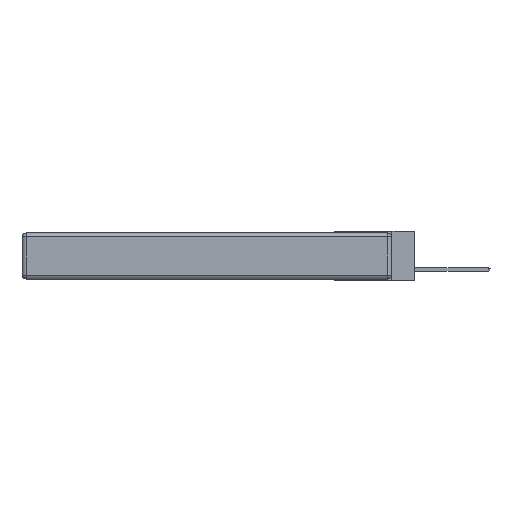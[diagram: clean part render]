
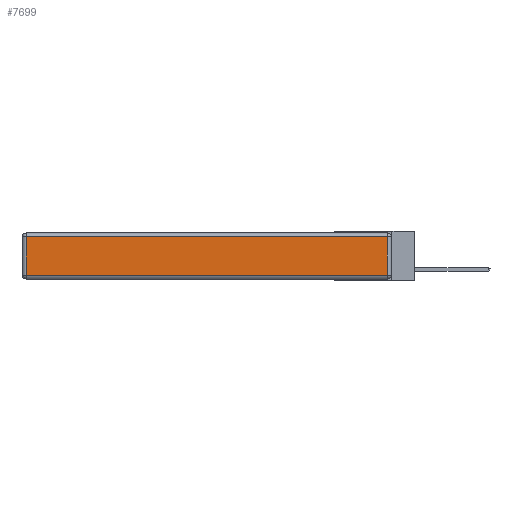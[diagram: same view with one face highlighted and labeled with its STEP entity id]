
A CAD part, left-side view. The second image highlights one B-rep face of the part: STEP entity #7699.
In plain terms, the highlighted planar face has unit normal (-1, 0, 0).
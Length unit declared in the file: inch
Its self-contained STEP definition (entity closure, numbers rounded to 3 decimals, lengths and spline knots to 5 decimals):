
#28 = VERTEX_POINT ( 'NONE', #29723 ) ;
#1536 = CARTESIAN_POINT ( 'NONE',  ( 0., 0.03, -0.313 ) ) ;
#2523 = EDGE_CURVE ( 'NONE', #28, #14178, #12513, .T. ) ;
#3996 = EDGE_CURVE ( 'NONE', #13400, #28, #24010, .T. ) ;
#4751 = CARTESIAN_POINT ( 'NONE',  ( 0., 0., -0.343 ) ) ;
#4895 = VECTOR ( 'NONE', #13165, 39.37008 ) ;
#5603 = VECTOR ( 'NONE', #11406, 39.37008 ) ;
#6457 = CARTESIAN_POINT ( 'NONE',  ( 0., 0.03, -0.343 ) ) ;
#7699 = ADVANCED_FACE ( 'NONE', ( #17677 ), #16324, .T. ) ;
#9104 = EDGE_CURVE ( 'NONE', #22002, #13400, #26489, .T. ) ;
#9257 = CARTESIAN_POINT ( 'NONE',  ( 0., 2.75, -0.03 ) ) ;
#10375 = ORIENTED_EDGE ( 'NONE', *, *, #22094, .T. ) ;
#11406 = DIRECTION ( 'NONE',  ( 0., 1., 0. ) ) ;
#12513 = LINE ( 'NONE', #18582, #19684 ) ;
#13165 = DIRECTION ( 'NONE',  ( 0., 0., 1. ) ) ;
#13400 = VERTEX_POINT ( 'NONE', #25980 ) ;
#14065 = ORIENTED_EDGE ( 'NONE', *, *, #2523, .T. ) ;
#14178 = VERTEX_POINT ( 'NONE', #20169 ) ;
#15516 = DIRECTION ( 'NONE',  ( 0., -1., 0. ) ) ;
#16324 = PLANE ( 'NONE',  #28177 ) ;
#16948 = ORIENTED_EDGE ( 'NONE', *, *, #9104, .T. ) ;
#17677 = FACE_OUTER_BOUND ( 'NONE', #24665, .T. ) ;
#18582 = CARTESIAN_POINT ( 'NONE',  ( 0., 2.72, -0.343 ) ) ;
#19485 = LINE ( 'NONE', #26911, #29149 ) ;
#19684 = VECTOR ( 'NONE', #20997, 39.37008 ) ;
#20169 = CARTESIAN_POINT ( 'NONE',  ( 0., 2.72, -0.313 ) ) ;
#20528 = DIRECTION ( 'NONE',  ( -1., 0., 0. ) ) ;
#20736 = DIRECTION ( 'NONE',  ( 0., 0., 1. ) ) ;
#20997 = DIRECTION ( 'NONE',  ( 0., 0., -1. ) ) ;
#22002 = VERTEX_POINT ( 'NONE', #1536 ) ;
#22094 = EDGE_CURVE ( 'NONE', #14178, #22002, #19485, .T. ) ;
#24010 = LINE ( 'NONE', #9257, #5603 ) ;
#24665 = EDGE_LOOP ( 'NONE', ( #10375, #16948, #27610, #14065 ) ) ;
#25980 = CARTESIAN_POINT ( 'NONE',  ( 0., 0.03, -0.03 ) ) ;
#26489 = LINE ( 'NONE', #6457, #4895 ) ;
#26911 = CARTESIAN_POINT ( 'NONE',  ( 0., 0., -0.313 ) ) ;
#27610 = ORIENTED_EDGE ( 'NONE', *, *, #3996, .T. ) ;
#28177 = AXIS2_PLACEMENT_3D ( 'NONE', #4751, #20528, #20736 ) ;
#29149 = VECTOR ( 'NONE', #15516, 39.37008 ) ;
#29723 = CARTESIAN_POINT ( 'NONE',  ( 0., 2.72, -0.03 ) ) ;
